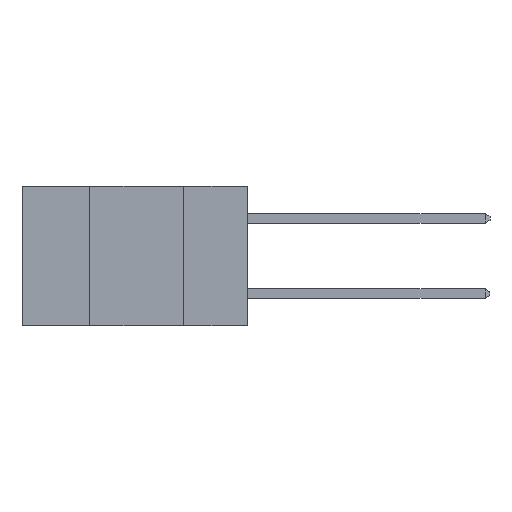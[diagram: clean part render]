
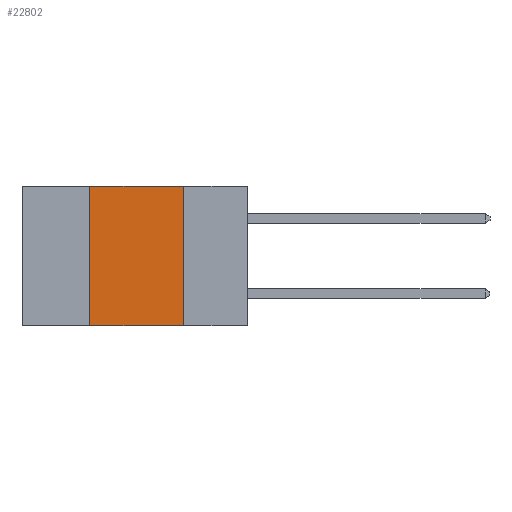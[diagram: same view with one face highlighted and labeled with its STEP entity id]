
A CAD part, left-side view. The second image highlights one B-rep face of the part: STEP entity #22802.
In plain terms, the highlighted planar face has unit normal (-1, 0, 0).
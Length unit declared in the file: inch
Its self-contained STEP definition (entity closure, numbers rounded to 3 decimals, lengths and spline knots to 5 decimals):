
#617 = VERTEX_POINT ( 'NONE', #10067 ) ;
#1146 = DIRECTION ( 'NONE',  ( 1., 0., 0. ) ) ;
#1589 = LINE ( 'NONE', #11468, #14223 ) ;
#1608 = DIRECTION ( 'NONE',  ( 0., -1., 0. ) ) ;
#3885 = ORIENTED_EDGE ( 'NONE', *, *, #19274, .F. ) ;
#5471 = ORIENTED_EDGE ( 'NONE', *, *, #12926, .F. ) ;
#5659 = VERTEX_POINT ( 'NONE', #31679 ) ;
#6097 = EDGE_LOOP ( 'NONE', ( #3885, #5471, #18846, #7043 ) ) ;
#6697 = CARTESIAN_POINT ( 'NONE',  ( 0., 0.6, 0. ) ) ;
#7043 = ORIENTED_EDGE ( 'NONE', *, *, #29863, .T. ) ;
#7636 = VECTOR ( 'NONE', #27298, 39.37008 ) ;
#7945 = VERTEX_POINT ( 'NONE', #10528 ) ;
#9736 = LINE ( 'NONE', #6697, #28256 ) ;
#10067 = CARTESIAN_POINT ( 'NONE',  ( 0., 0.42, -0.37 ) ) ;
#10528 = CARTESIAN_POINT ( 'NONE',  ( 0., 0.17, -0.37 ) ) ;
#10858 = AXIS2_PLACEMENT_3D ( 'NONE', #31335, #1146, #18760 ) ;
#11468 = CARTESIAN_POINT ( 'NONE',  ( 0., 0.6, -0.37 ) ) ;
#12926 = EDGE_CURVE ( 'NONE', #16020, #5659, #9736, .T. ) ;
#13445 = CARTESIAN_POINT ( 'NONE',  ( 0., 0.17, 0. ) ) ;
#14016 = DIRECTION ( 'NONE',  ( 0., -1., 0. ) ) ;
#14223 = VECTOR ( 'NONE', #14016, 39.37008 ) ;
#16020 = VERTEX_POINT ( 'NONE', #20316 ) ;
#17096 = LINE ( 'NONE', #13445, #29733 ) ;
#18760 = DIRECTION ( 'NONE',  ( 0., 0., -1. ) ) ;
#18846 = ORIENTED_EDGE ( 'NONE', *, *, #28130, .F. ) ;
#19274 = EDGE_CURVE ( 'NONE', #5659, #7945, #17096, .T. ) ;
#20316 = CARTESIAN_POINT ( 'NONE',  ( 0., 0.42, 0. ) ) ;
#22802 = ADVANCED_FACE ( 'NONE', ( #27186 ), #28825, .F. ) ;
#27186 = FACE_OUTER_BOUND ( 'NONE', #6097, .T. ) ;
#27298 = DIRECTION ( 'NONE',  ( 0., 0., 1. ) ) ;
#27732 = LINE ( 'NONE', #29842, #7636 ) ;
#28130 = EDGE_CURVE ( 'NONE', #617, #16020, #27732, .T. ) ;
#28256 = VECTOR ( 'NONE', #1608, 39.37008 ) ;
#28524 = DIRECTION ( 'NONE',  ( 0., 0., -1. ) ) ;
#28825 = PLANE ( 'NONE',  #10858 ) ;
#29733 = VECTOR ( 'NONE', #28524, 39.37008 ) ;
#29842 = CARTESIAN_POINT ( 'NONE',  ( 0., 0.42, 0. ) ) ;
#29863 = EDGE_CURVE ( 'NONE', #617, #7945, #1589, .T. ) ;
#31335 = CARTESIAN_POINT ( 'NONE',  ( 0., 0.6, 0. ) ) ;
#31679 = CARTESIAN_POINT ( 'NONE',  ( 0., 0.17, 0. ) ) ;
